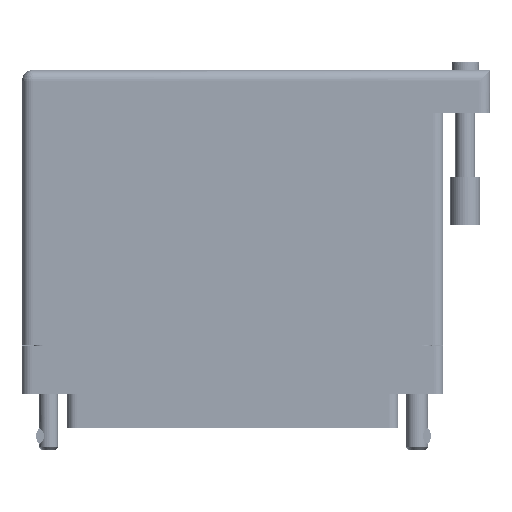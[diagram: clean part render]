
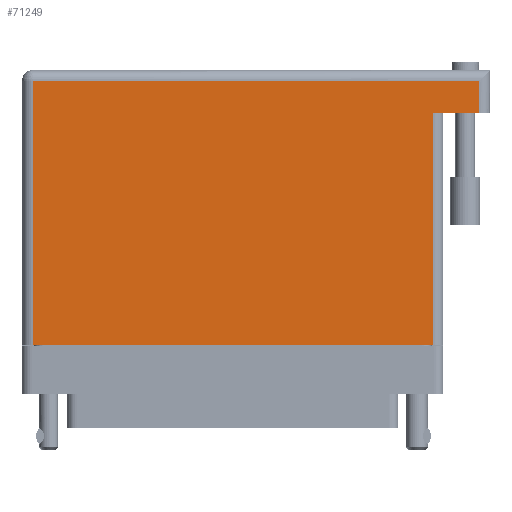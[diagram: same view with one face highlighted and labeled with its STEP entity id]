
A CAD part, front view. The second image highlights one B-rep face of the part: STEP entity #71249.
In plain terms, the highlighted face is planar.
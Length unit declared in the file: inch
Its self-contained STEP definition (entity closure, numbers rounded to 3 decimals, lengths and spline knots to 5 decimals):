
#84 = ORIENTED_EDGE ( 'NONE', *, *, #36743, .F. ) ;
#1492 = VECTOR ( 'NONE', #29474, 39.37008 ) ;
#1727 = CARTESIAN_POINT ( 'NONE',  ( 1.659, 1.395, 0.617 ) ) ;
#2142 = LINE ( 'NONE', #6303, #69910 ) ;
#2361 = EDGE_CURVE ( 'NONE', #38151, #60437, #78733, .T. ) ;
#3330 = AXIS2_PLACEMENT_3D ( 'NONE', #83075, #57671, #18912 ) ;
#5274 = CARTESIAN_POINT ( 'NONE',  ( 1.289, -0.1, 0.617 ) ) ;
#5870 = CARTESIAN_POINT ( 'NONE',  ( -1.289, 1.605, 0.617 ) ) ;
#6223 = CARTESIAN_POINT ( 'NONE',  ( -1.289, -0.1, 0.617 ) ) ;
#6303 = CARTESIAN_POINT ( 'NONE',  ( 1.589, 1.675, 0.617 ) ) ;
#7995 = DIRECTION ( 'NONE',  ( 0., 1., 0. ) ) ;
#9787 = CARTESIAN_POINT ( 'NONE',  ( 1.589, 1.605, 0.617 ) ) ;
#10575 = ORIENTED_EDGE ( 'NONE', *, *, #2361, .T. ) ;
#12975 = ORIENTED_EDGE ( 'NONE', *, *, #69516, .T. ) ;
#13793 = DIRECTION ( 'NONE',  ( -1., 0., 0. ) ) ;
#16074 = FACE_OUTER_BOUND ( 'NONE', #22043, .T. ) ;
#17843 = ORIENTED_EDGE ( 'NONE', *, *, #22225, .T. ) ;
#18912 = DIRECTION ( 'NONE',  ( -1., 0., 0. ) ) ;
#19149 = CARTESIAN_POINT ( 'NONE',  ( -1.359, -0.1, 0.617 ) ) ;
#22043 = EDGE_LOOP ( 'NONE', ( #10575, #55880, #84, #12975, #57347, #17843 ) ) ;
#22225 = EDGE_CURVE ( 'NONE', #53814, #38151, #30290, .T. ) ;
#28915 = LINE ( 'NONE', #1727, #1492 ) ;
#29474 = DIRECTION ( 'NONE',  ( -1., 0., 0. ) ) ;
#30290 = LINE ( 'NONE', #6223, #71724 ) ;
#30783 = VERTEX_POINT ( 'NONE', #39587 ) ;
#32890 = LINE ( 'NONE', #78899, #76247 ) ;
#33588 = VECTOR ( 'NONE', #13793, 39.37008 ) ;
#36743 = EDGE_CURVE ( 'NONE', #30783, #66822, #28915, .T. ) ;
#38151 = VERTEX_POINT ( 'NONE', #77661 ) ;
#39587 = CARTESIAN_POINT ( 'NONE',  ( 1.589, 1.395, 0.617 ) ) ;
#42343 = VECTOR ( 'NONE', #57364, 39.37008 ) ;
#43662 = LINE ( 'NONE', #59031, #33588 ) ;
#53814 = VERTEX_POINT ( 'NONE', #5870 ) ;
#55880 = ORIENTED_EDGE ( 'NONE', *, *, #74112, .T. ) ;
#57347 = ORIENTED_EDGE ( 'NONE', *, *, #57977, .T. ) ;
#57364 = DIRECTION ( 'NONE',  ( 1., 0., 0. ) ) ;
#57671 = DIRECTION ( 'NONE',  ( 0., 0., -1. ) ) ;
#57970 = DIRECTION ( 'NONE',  ( 0., -1., 0. ) ) ;
#57977 = EDGE_CURVE ( 'NONE', #68936, #53814, #43662, .T. ) ;
#59031 = CARTESIAN_POINT ( 'NONE',  ( -1.359, 1.605, 0.617 ) ) ;
#60437 = VERTEX_POINT ( 'NONE', #5274 ) ;
#64527 = DIRECTION ( 'NONE',  ( 0., 1., 0. ) ) ;
#66822 = VERTEX_POINT ( 'NONE', #76569 ) ;
#68936 = VERTEX_POINT ( 'NONE', #9787 ) ;
#69516 = EDGE_CURVE ( 'NONE', #30783, #68936, #2142, .T. ) ;
#69910 = VECTOR ( 'NONE', #64527, 39.37008 ) ;
#71249 = ADVANCED_FACE ( 'NONE', ( #16074 ), #76817, .F. ) ;
#71724 = VECTOR ( 'NONE', #57970, 39.37008 ) ;
#74112 = EDGE_CURVE ( 'NONE', #60437, #66822, #32890, .T. ) ;
#76247 = VECTOR ( 'NONE', #7995, 39.37008 ) ;
#76569 = CARTESIAN_POINT ( 'NONE',  ( 1.289, 1.395, 0.617 ) ) ;
#76817 = PLANE ( 'NONE',  #3330 ) ;
#77661 = CARTESIAN_POINT ( 'NONE',  ( -1.289, -0.1, 0.617 ) ) ;
#78733 = LINE ( 'NONE', #19149, #42343 ) ;
#78899 = CARTESIAN_POINT ( 'NONE',  ( 1.289, 1.395, 0.617 ) ) ;
#83075 = CARTESIAN_POINT ( 'NONE',  ( -1.359, 1.675, 0.617 ) ) ;
